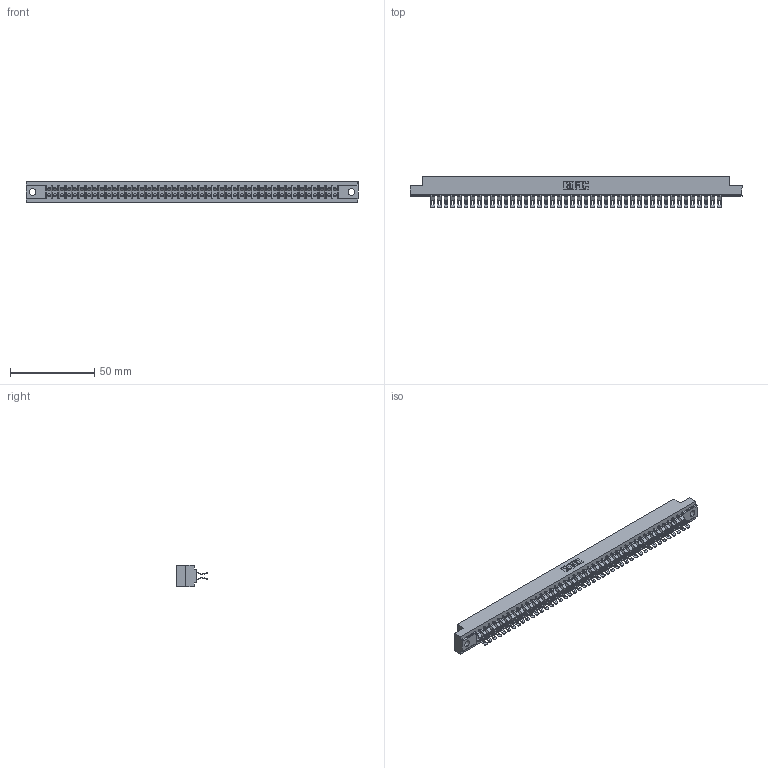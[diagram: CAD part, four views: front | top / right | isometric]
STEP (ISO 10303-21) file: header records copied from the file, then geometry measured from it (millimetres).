
FILE_DESCRIPTION (( 'STEP AP203' ), '1' );
FILE_NAME ('807-088-555-204.STEP', '2021-07-20T21:11:55', ( '' ), ( '' ), 'SwSTEP 2.0', 'SolidWorks 2020', '' );
FILE_SCHEMA (( 'CONFIG_CONTROL_DESIGN' ));
Length unit declared in the file: inch
Products named in the file (3): 807 Part_.156 Dia Mounting Holes; 807-088-555-204; 307-290-001_555
Assembly tree (89 placements, depth 2):
  807-088-555-204
    807 Part_.156 Dia Mounting Holes
    307-290-001_555  x88
Bounding box: 197.36 x 18.75 x 12.7 mm (x, y, z)
Volume: 21157.1 mm3; surface area: 27216 mm2
Topology: 89 solids, 89 shells, 5545 faces, 16287 edges, 10618 vertices
Faces by surface type: plane 3076, cylinder 2379, sphere 90
Entity records: 39837 total; most frequent: CARTESIAN_POINT 6526, ORIENTED_EDGE 6468, DIRECTION 6390, EDGE_CURVE 3234, LINE 2478, VECTOR 2478, VERTEX_POINT 2092, AXIS2_PLACEMENT_3D 1956
